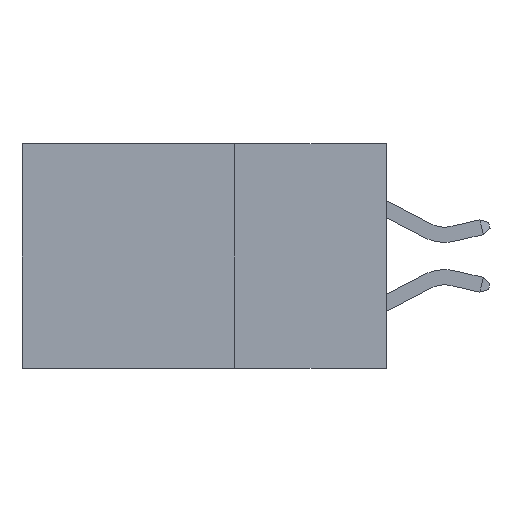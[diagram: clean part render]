
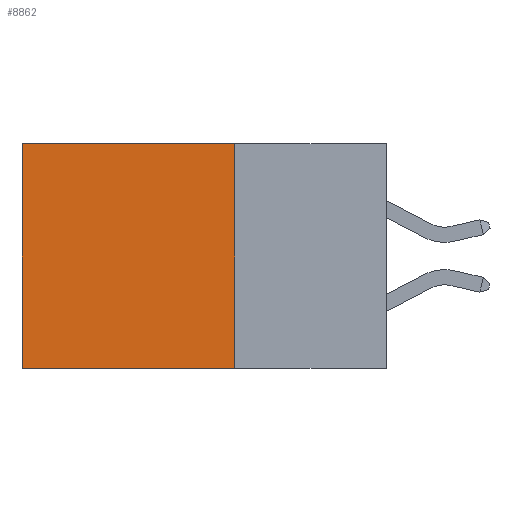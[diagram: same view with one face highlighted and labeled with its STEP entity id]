
A CAD part, left-side view. The second image highlights one B-rep face of the part: STEP entity #8862.
In plain terms, the highlighted planar face has unit normal (-1, 0, 0).
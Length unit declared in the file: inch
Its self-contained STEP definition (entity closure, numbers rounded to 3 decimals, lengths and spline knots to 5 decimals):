
#617 = PLANE ( 'NONE',  #11059 ) ;
#800 = VECTOR ( 'NONE', #13804, 39.37008 ) ;
#860 = EDGE_CURVE ( 'NONE', #16778, #1660, #3225, .T. ) ;
#1660 = VERTEX_POINT ( 'NONE', #15382 ) ;
#1954 = CARTESIAN_POINT ( 'NONE',  ( 0.2615, 0.25, -0.37 ) ) ;
#2419 = VERTEX_POINT ( 'NONE', #12246 ) ;
#2734 = CARTESIAN_POINT ( 'NONE',  ( 0.2615, 0.6, 0. ) ) ;
#3225 = LINE ( 'NONE', #4385, #16339 ) ;
#3568 = ORIENTED_EDGE ( 'NONE', *, *, #11992, .F. ) ;
#3627 = CARTESIAN_POINT ( 'NONE',  ( 0.2615, 0.6, -0.37 ) ) ;
#4385 = CARTESIAN_POINT ( 'NONE',  ( 0.2615, 0.25, -0.37 ) ) ;
#4698 = DIRECTION ( 'NONE',  ( 0., 0., -1. ) ) ;
#5404 = LINE ( 'NONE', #10798, #800 ) ;
#5444 = LINE ( 'NONE', #10837, #9782 ) ;
#5808 = ORIENTED_EDGE ( 'NONE', *, *, #860, .F. ) ;
#5936 = FACE_OUTER_BOUND ( 'NONE', #17262, .T. ) ;
#6202 = DIRECTION ( 'NONE',  ( 1., 0., 0. ) ) ;
#6347 = ORIENTED_EDGE ( 'NONE', *, *, #17477, .T. ) ;
#8862 = ADVANCED_FACE ( 'NONE', ( #5936 ), #617, .F. ) ;
#9377 = DIRECTION ( 'NONE',  ( 0., 0., -1. ) ) ;
#9782 = VECTOR ( 'NONE', #16239, 39.37008 ) ;
#10554 = ORIENTED_EDGE ( 'NONE', *, *, #16720, .T. ) ;
#10798 = CARTESIAN_POINT ( 'NONE',  ( 0.2615, 0.25, -0.37 ) ) ;
#10837 = CARTESIAN_POINT ( 'NONE',  ( 0.2615, 0.25, 0. ) ) ;
#11059 = AXIS2_PLACEMENT_3D ( 'NONE', #1954, #6202, #4698 ) ;
#11532 = CARTESIAN_POINT ( 'NONE',  ( 0.2615, 0.25, 0. ) ) ;
#11992 = EDGE_CURVE ( 'NONE', #1660, #2419, #5404, .T. ) ;
#12052 = VERTEX_POINT ( 'NONE', #2734 ) ;
#12246 = CARTESIAN_POINT ( 'NONE',  ( 0.2615, 0.6, -0.37 ) ) ;
#13804 = DIRECTION ( 'NONE',  ( 0., 1., 0. ) ) ;
#15174 = DIRECTION ( 'NONE',  ( 0., 0., -1. ) ) ;
#15382 = CARTESIAN_POINT ( 'NONE',  ( 0.2615, 0.25, -0.37 ) ) ;
#15753 = LINE ( 'NONE', #3627, #16270 ) ;
#16239 = DIRECTION ( 'NONE',  ( 0., 1., 0. ) ) ;
#16270 = VECTOR ( 'NONE', #9377, 39.37008 ) ;
#16339 = VECTOR ( 'NONE', #15174, 39.37008 ) ;
#16720 = EDGE_CURVE ( 'NONE', #16778, #12052, #5444, .T. ) ;
#16778 = VERTEX_POINT ( 'NONE', #11532 ) ;
#17262 = EDGE_LOOP ( 'NONE', ( #6347, #3568, #5808, #10554 ) ) ;
#17477 = EDGE_CURVE ( 'NONE', #12052, #2419, #15753, .T. ) ;
